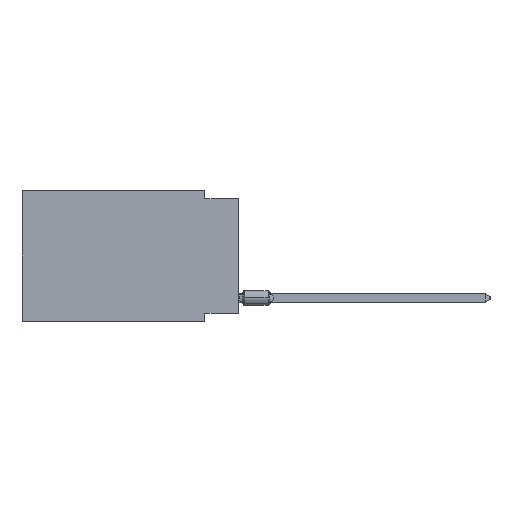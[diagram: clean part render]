
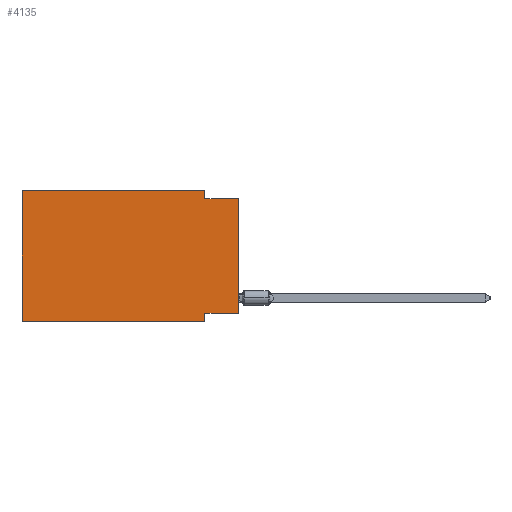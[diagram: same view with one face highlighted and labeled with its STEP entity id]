
A CAD part, left-side view. The second image highlights one B-rep face of the part: STEP entity #4135.
In plain terms, the highlighted planar face has unit normal (-1, 0, 0).
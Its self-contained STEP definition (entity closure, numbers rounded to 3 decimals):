
#628 = AXIS2_PLACEMENT_3D ( 'NONE', #51766, #42858, #19556 ) ;
#679 = VERTEX_POINT ( 'NONE', #28569 ) ;
#800 = PLANE ( 'NONE',  #628 ) ;
#3345 = LINE ( 'NONE', #11973, #4558 ) ;
#4135 = ADVANCED_FACE ( 'NONE', ( #33070 ), #800, .F. ) ;
#4558 = VECTOR ( 'NONE', #40197, 1000. ) ;
#5925 = DIRECTION ( 'NONE',  ( 0., -1., 0. ) ) ;
#6954 = VERTEX_POINT ( 'NONE', #32116 ) ;
#7954 = LINE ( 'NONE', #35300, #27667 ) ;
#8209 = CARTESIAN_POINT ( 'NONE',  ( 0., 0., 0. ) ) ;
#9783 = ORIENTED_EDGE ( 'NONE', *, *, #38013, .F. ) ;
#10879 = DIRECTION ( 'NONE',  ( 0., 1., 0. ) ) ;
#10975 = EDGE_CURVE ( 'NONE', #51005, #14371, #38272, .T. ) ;
#11207 = VECTOR ( 'NONE', #5925, 1000. ) ;
#11213 = CARTESIAN_POINT ( 'NONE',  ( 0., 2.54, 0. ) ) ;
#11608 = CARTESIAN_POINT ( 'NONE',  ( 0., 16.383, 0. ) ) ;
#11973 = CARTESIAN_POINT ( 'NONE',  ( 0., 2.54, -9.906 ) ) ;
#12295 = CARTESIAN_POINT ( 'NONE',  ( 0., 16.383, 0. ) ) ;
#12510 = DIRECTION ( 'NONE',  ( 0., 0., 1. ) ) ;
#13316 = CARTESIAN_POINT ( 'NONE',  ( 0., 2.54, -9.271 ) ) ;
#13632 = ORIENTED_EDGE ( 'NONE', *, *, #20221, .F. ) ;
#14155 = VECTOR ( 'NONE', #10879, 1000. ) ;
#14371 = VERTEX_POINT ( 'NONE', #30885 ) ;
#14560 = VECTOR ( 'NONE', #40826, 1000. ) ;
#14849 = ORIENTED_EDGE ( 'NONE', *, *, #59540, .F. ) ;
#14960 = CARTESIAN_POINT ( 'NONE',  ( 0., 2.54, 0. ) ) ;
#15824 = EDGE_CURVE ( 'NONE', #18811, #22834, #40439, .T. ) ;
#17211 = VECTOR ( 'NONE', #12510, 1000. ) ;
#17586 = EDGE_CURVE ( 'NONE', #679, #51005, #21504, .T. ) ;
#18811 = VERTEX_POINT ( 'NONE', #47148 ) ;
#19556 = DIRECTION ( 'NONE',  ( 0., 0., -1. ) ) ;
#20221 = EDGE_CURVE ( 'NONE', #6954, #679, #30355, .T. ) ;
#20531 = ORIENTED_EDGE ( 'NONE', *, *, #15824, .T. ) ;
#21504 = LINE ( 'NONE', #12295, #14560 ) ;
#21620 = LINE ( 'NONE', #48294, #14155 ) ;
#22204 = VERTEX_POINT ( 'NONE', #43976 ) ;
#22834 = VERTEX_POINT ( 'NONE', #32981 ) ;
#22949 = EDGE_CURVE ( 'NONE', #14371, #22834, #38176, .T. ) ;
#24794 = EDGE_LOOP ( 'NONE', ( #20531, #58827, #60422, #28909, #13632, #53371, #14849, #9783 ) ) ;
#25738 = DIRECTION ( 'NONE',  ( 0., 0., 1. ) ) ;
#26689 = DIRECTION ( 'NONE',  ( 0., -1., 0. ) ) ;
#27667 = VECTOR ( 'NONE', #26689, 1000. ) ;
#28362 = VECTOR ( 'NONE', #25738, 1000. ) ;
#28569 = CARTESIAN_POINT ( 'NONE',  ( 0., 16.383, 0. ) ) ;
#28780 = DIRECTION ( 'NONE',  ( 0., 0., -1. ) ) ;
#28909 = ORIENTED_EDGE ( 'NONE', *, *, #17586, .F. ) ;
#30355 = LINE ( 'NONE', #11608, #28362 ) ;
#30885 = CARTESIAN_POINT ( 'NONE',  ( 0., 2.54, -0.635 ) ) ;
#31815 = EDGE_CURVE ( 'NONE', #6954, #22204, #7954, .T. ) ;
#32116 = CARTESIAN_POINT ( 'NONE',  ( 0., 16.383, -9.906 ) ) ;
#32981 = CARTESIAN_POINT ( 'NONE',  ( 0., 0., -0.635 ) ) ;
#33070 = FACE_OUTER_BOUND ( 'NONE', #24794, .T. ) ;
#34488 = CARTESIAN_POINT ( 'NONE',  ( 0., 0., -0.635 ) ) ;
#35300 = CARTESIAN_POINT ( 'NONE',  ( 0., 16.383, -9.906 ) ) ;
#38013 = EDGE_CURVE ( 'NONE', #18811, #39941, #21620, .T. ) ;
#38176 = LINE ( 'NONE', #34488, #11207 ) ;
#38272 = LINE ( 'NONE', #14960, #53194 ) ;
#39941 = VERTEX_POINT ( 'NONE', #13316 ) ;
#40197 = DIRECTION ( 'NONE',  ( 0., 0., -1. ) ) ;
#40439 = LINE ( 'NONE', #8209, #17211 ) ;
#40826 = DIRECTION ( 'NONE',  ( 0., -1., 0. ) ) ;
#42858 = DIRECTION ( 'NONE',  ( 1., 0., 0. ) ) ;
#43976 = CARTESIAN_POINT ( 'NONE',  ( 0., 2.54, -9.906 ) ) ;
#47148 = CARTESIAN_POINT ( 'NONE',  ( 0., 0., -9.271 ) ) ;
#48294 = CARTESIAN_POINT ( 'NONE',  ( 0., 0., -9.271 ) ) ;
#51005 = VERTEX_POINT ( 'NONE', #11213 ) ;
#51766 = CARTESIAN_POINT ( 'NONE',  ( 0., 16.383, 0. ) ) ;
#53194 = VECTOR ( 'NONE', #28780, 1000. ) ;
#53371 = ORIENTED_EDGE ( 'NONE', *, *, #31815, .T. ) ;
#58827 = ORIENTED_EDGE ( 'NONE', *, *, #22949, .F. ) ;
#59540 = EDGE_CURVE ( 'NONE', #39941, #22204, #3345, .T. ) ;
#60422 = ORIENTED_EDGE ( 'NONE', *, *, #10975, .F. ) ;
